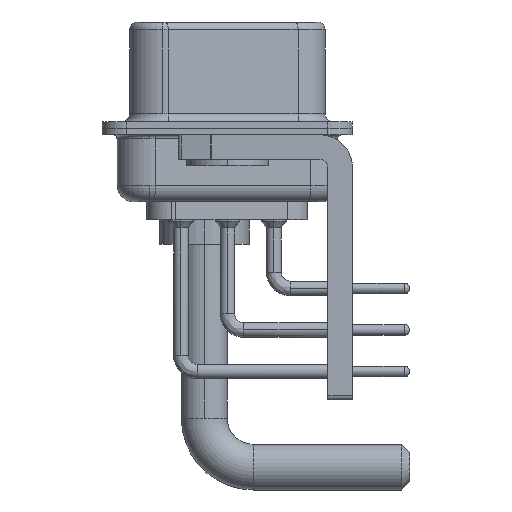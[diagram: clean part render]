
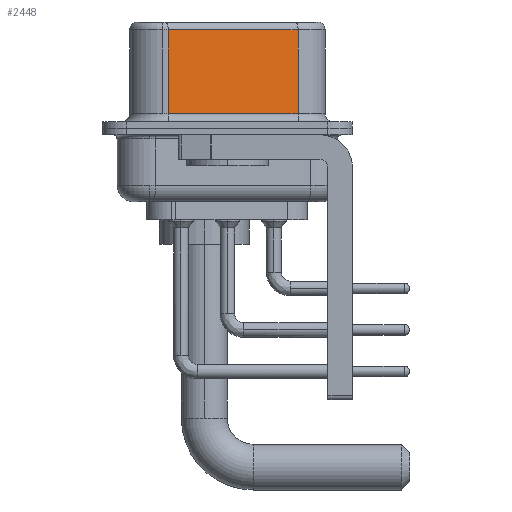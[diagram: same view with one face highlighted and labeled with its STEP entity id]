
A CAD part, left-side view. The second image highlights one B-rep face of the part: STEP entity #2448.
In plain terms, the highlighted planar face has unit normal (-0.985, -0.174, 0).
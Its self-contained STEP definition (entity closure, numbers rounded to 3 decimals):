
#1326 = EDGE_CURVE ( 'NONE', #33928, #14825, #14163, .T. ) ;
#2448 = ADVANCED_FACE ( 'NONE', ( #24967 ), #30409, .F. ) ;
#2925 = EDGE_CURVE ( 'NONE', #14825, #18328, #24921, .T. ) ;
#3758 = DIRECTION ( 'NONE',  ( -0.174, 0.985, 0. ) ) ;
#4198 = VERTEX_POINT ( 'NONE', #23394 ) ;
#5861 = DIRECTION ( 'NONE',  ( -0.174, 0.985, 0. ) ) ;
#7349 = DIRECTION ( 'NONE',  ( 0., 0., -1. ) ) ;
#7811 = CARTESIAN_POINT ( 'NONE',  ( 3.73, 3.628, 0.9 ) ) ;
#7818 = VECTOR ( 'NONE', #7349, 1000. ) ;
#7948 = VECTOR ( 'NONE', #36719, 1000. ) ;
#8279 = LINE ( 'NONE', #30575, #27573 ) ;
#10792 = ORIENTED_EDGE ( 'NONE', *, *, #2925, .T. ) ;
#11163 = DIRECTION ( 'NONE',  ( 0., 0., -1. ) ) ;
#14163 = LINE ( 'NONE', #14360, #25031 ) ;
#14360 = CARTESIAN_POINT ( 'NONE',  ( 5.132, -4.322, 6.02 ) ) ;
#14825 = VERTEX_POINT ( 'NONE', #31275 ) ;
#16952 = ORIENTED_EDGE ( 'NONE', *, *, #37437, .T. ) ;
#18328 = VERTEX_POINT ( 'NONE', #7811 ) ;
#18379 = ORIENTED_EDGE ( 'NONE', *, *, #29120, .F. ) ;
#18771 = LINE ( 'NONE', #21483, #7948 ) ;
#21333 = DIRECTION ( 'NONE',  ( 0.985, 0.174, 0. ) ) ;
#21483 = CARTESIAN_POINT ( 'NONE',  ( 5.132, -4.322, 0.9 ) ) ;
#22259 = CARTESIAN_POINT ( 'NONE',  ( 5.132, -4.322, 6.02 ) ) ;
#23394 = CARTESIAN_POINT ( 'NONE',  ( 5.132, -4.322, 0.9 ) ) ;
#24921 = LINE ( 'NONE', #36704, #7818 ) ;
#24967 = FACE_OUTER_BOUND ( 'NONE', #25124, .T. ) ;
#25031 = VECTOR ( 'NONE', #5861, 1000. ) ;
#25124 = EDGE_LOOP ( 'NONE', ( #18379, #31614, #10792, #16952 ) ) ;
#26924 = AXIS2_PLACEMENT_3D ( 'NONE', #30969, #21333, #3758 ) ;
#27573 = VECTOR ( 'NONE', #11163, 1000. ) ;
#29120 = EDGE_CURVE ( 'NONE', #33928, #4198, #8279, .T. ) ;
#30409 = PLANE ( 'NONE',  #26924 ) ;
#30575 = CARTESIAN_POINT ( 'NONE',  ( 5.132, -4.322, 6.52 ) ) ;
#30969 = CARTESIAN_POINT ( 'NONE',  ( 5.132, -4.322, 6.52 ) ) ;
#31275 = CARTESIAN_POINT ( 'NONE',  ( 3.73, 3.628, 6.02 ) ) ;
#31614 = ORIENTED_EDGE ( 'NONE', *, *, #1326, .T. ) ;
#33928 = VERTEX_POINT ( 'NONE', #22259 ) ;
#36704 = CARTESIAN_POINT ( 'NONE',  ( 3.73, 3.628, 6.52 ) ) ;
#36719 = DIRECTION ( 'NONE',  ( 0.174, -0.985, 0. ) ) ;
#37437 = EDGE_CURVE ( 'NONE', #18328, #4198, #18771, .T. ) ;
